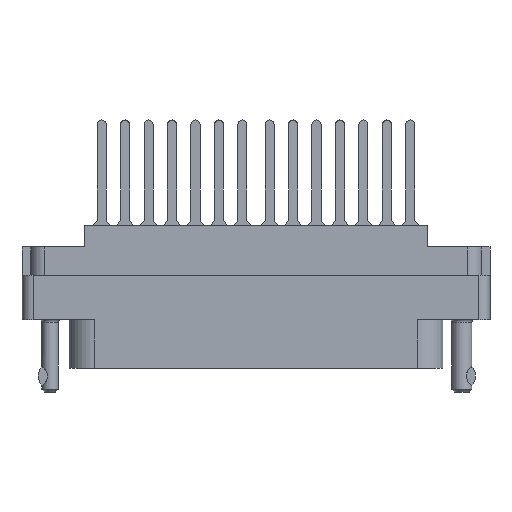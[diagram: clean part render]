
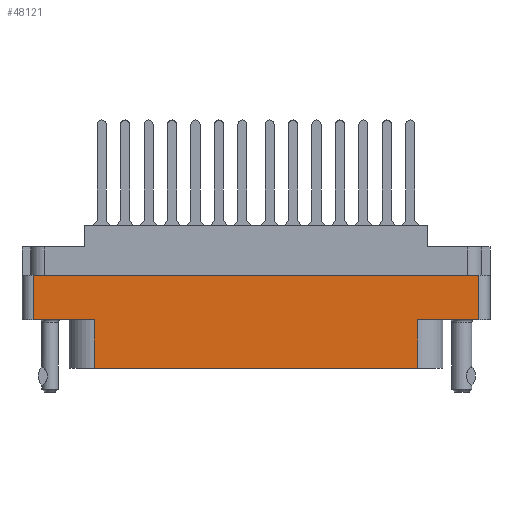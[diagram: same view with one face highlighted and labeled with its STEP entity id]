
A CAD part, front view. The second image highlights one B-rep face of the part: STEP entity #48121.
In plain terms, the highlighted planar face has unit normal (0, -1, 0).
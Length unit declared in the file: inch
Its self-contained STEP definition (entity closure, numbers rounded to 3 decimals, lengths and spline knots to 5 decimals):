
#369 = VECTOR ( 'NONE', #55750, 39.37008 ) ;
#1835 = VERTEX_POINT ( 'NONE', #35242 ) ;
#1901 = VECTOR ( 'NONE', #26830, 39.37008 ) ;
#2638 = LINE ( 'NONE', #35541, #49417 ) ;
#5984 = EDGE_CURVE ( 'NONE', #21511, #39820, #42929, .T. ) ;
#6166 = PLANE ( 'NONE',  #21037 ) ;
#6511 = LINE ( 'NONE', #11491, #55365 ) ;
#10332 = CARTESIAN_POINT ( 'NONE',  ( 0.895, -0.438, -0.789 ) ) ;
#11491 = CARTESIAN_POINT ( 'NONE',  ( 1.2335, -0.438, -0.789 ) ) ;
#11564 = CARTESIAN_POINT ( 'NONE',  ( 1.2335, -0.438, -0.274 ) ) ;
#13446 = CARTESIAN_POINT ( 'NONE',  ( 0.895, -0.438, -0.52 ) ) ;
#14829 = VECTOR ( 'NONE', #19122, 39.37008 ) ;
#15077 = CARTESIAN_POINT ( 'NONE',  ( -0.895, -0.438, -0.789 ) ) ;
#15096 = DIRECTION ( 'NONE',  ( -1., 0., 0. ) ) ;
#15471 = EDGE_CURVE ( 'NONE', #56596, #58406, #6511, .T. ) ;
#17830 = DIRECTION ( 'NONE',  ( 1., 0., 0. ) ) ;
#18071 = ORIENTED_EDGE ( 'NONE', *, *, #31147, .F. ) ;
#18310 = ORIENTED_EDGE ( 'NONE', *, *, #57945, .F. ) ;
#19122 = DIRECTION ( 'NONE',  ( 0., 0., -1. ) ) ;
#19738 = DIRECTION ( 'NONE',  ( 0., -1., 0. ) ) ;
#20118 = DIRECTION ( 'NONE',  ( 0., 0., -1. ) ) ;
#21016 = EDGE_LOOP ( 'NONE', ( #18310, #55383, #45687, #55832, #26675, #23553, #18071, #39504 ) ) ;
#21037 = AXIS2_PLACEMENT_3D ( 'NONE', #28834, #19738, #20118 ) ;
#21511 = VERTEX_POINT ( 'NONE', #30152 ) ;
#21590 = CARTESIAN_POINT ( 'NONE',  ( 1.2335, -0.438, -0.52 ) ) ;
#23290 = LINE ( 'NONE', #46273, #14829 ) ;
#23396 = VECTOR ( 'NONE', #15096, 39.37008 ) ;
#23553 = ORIENTED_EDGE ( 'NONE', *, *, #33182, .T. ) ;
#24413 = LINE ( 'NONE', #15077, #369 ) ;
#24818 = LINE ( 'NONE', #46660, #23396 ) ;
#26675 = ORIENTED_EDGE ( 'NONE', *, *, #44892, .T. ) ;
#26792 = VERTEX_POINT ( 'NONE', #49000 ) ;
#26830 = DIRECTION ( 'NONE',  ( -1., 0., 0. ) ) ;
#28280 = LINE ( 'NONE', #45183, #46751 ) ;
#28834 = CARTESIAN_POINT ( 'NONE',  ( -1.2955, -0.438, -0.789 ) ) ;
#30152 = CARTESIAN_POINT ( 'NONE',  ( -0.895, -0.438, -0.52 ) ) ;
#30609 = CARTESIAN_POINT ( 'NONE',  ( -1.2335, -0.438, -0.52 ) ) ;
#31066 = VECTOR ( 'NONE', #45700, 39.37008 ) ;
#31147 = EDGE_CURVE ( 'NONE', #56596, #1835, #24818, .T. ) ;
#33182 = EDGE_CURVE ( 'NONE', #34623, #1835, #55240, .T. ) ;
#34623 = VERTEX_POINT ( 'NONE', #10332 ) ;
#35157 = CARTESIAN_POINT ( 'NONE',  ( 0., -0.438, -0.52 ) ) ;
#35242 = CARTESIAN_POINT ( 'NONE',  ( 0.895, -0.438, -0.52 ) ) ;
#35541 = CARTESIAN_POINT ( 'NONE',  ( 0., -0.438, -0.274 ) ) ;
#36611 = EDGE_CURVE ( 'NONE', #21511, #40286, #24413, .T. ) ;
#39504 = ORIENTED_EDGE ( 'NONE', *, *, #15471, .T. ) ;
#39820 = VERTEX_POINT ( 'NONE', #30609 ) ;
#40286 = VERTEX_POINT ( 'NONE', #51277 ) ;
#42929 = LINE ( 'NONE', #35157, #1901 ) ;
#44892 = EDGE_CURVE ( 'NONE', #40286, #34623, #28280, .T. ) ;
#45183 = CARTESIAN_POINT ( 'NONE',  ( -1.2955, -0.438, -0.789 ) ) ;
#45687 = ORIENTED_EDGE ( 'NONE', *, *, #5984, .F. ) ;
#45700 = DIRECTION ( 'NONE',  ( 0., 0., 1. ) ) ;
#46273 = CARTESIAN_POINT ( 'NONE',  ( -1.2335, -0.438, -0.789 ) ) ;
#46660 = CARTESIAN_POINT ( 'NONE',  ( 0., -0.438, -0.52 ) ) ;
#46751 = VECTOR ( 'NONE', #17830, 39.37008 ) ;
#48121 = ADVANCED_FACE ( 'NONE', ( #50617 ), #6166, .T. ) ;
#49000 = CARTESIAN_POINT ( 'NONE',  ( -1.2335, -0.438, -0.274 ) ) ;
#49417 = VECTOR ( 'NONE', #49863, 39.37008 ) ;
#49863 = DIRECTION ( 'NONE',  ( 1., 0., 0. ) ) ;
#50617 = FACE_OUTER_BOUND ( 'NONE', #21016, .T. ) ;
#51277 = CARTESIAN_POINT ( 'NONE',  ( -0.895, -0.438, -0.789 ) ) ;
#52229 = EDGE_CURVE ( 'NONE', #26792, #39820, #23290, .T. ) ;
#55240 = LINE ( 'NONE', #13446, #31066 ) ;
#55365 = VECTOR ( 'NONE', #56663, 39.37008 ) ;
#55383 = ORIENTED_EDGE ( 'NONE', *, *, #52229, .T. ) ;
#55750 = DIRECTION ( 'NONE',  ( 0., 0., -1. ) ) ;
#55832 = ORIENTED_EDGE ( 'NONE', *, *, #36611, .T. ) ;
#56596 = VERTEX_POINT ( 'NONE', #21590 ) ;
#56663 = DIRECTION ( 'NONE',  ( 0., 0., 1. ) ) ;
#57945 = EDGE_CURVE ( 'NONE', #26792, #58406, #2638, .T. ) ;
#58406 = VERTEX_POINT ( 'NONE', #11564 ) ;
